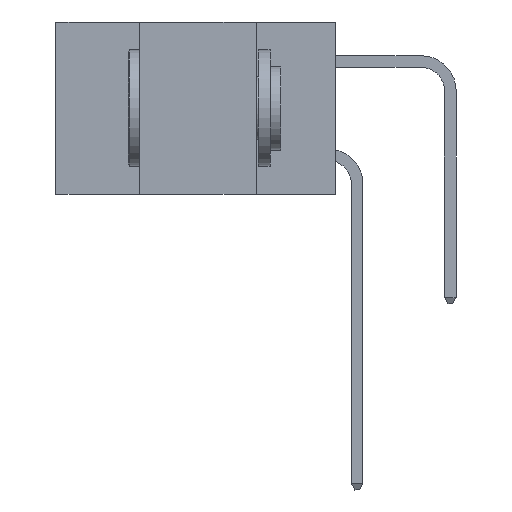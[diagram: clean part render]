
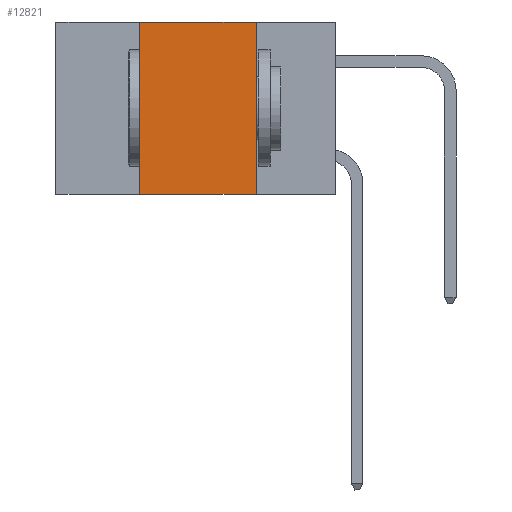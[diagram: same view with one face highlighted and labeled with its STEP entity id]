
A CAD part, left-side view. The second image highlights one B-rep face of the part: STEP entity #12821.
In plain terms, the highlighted planar face has unit normal (-1, 0, 0).
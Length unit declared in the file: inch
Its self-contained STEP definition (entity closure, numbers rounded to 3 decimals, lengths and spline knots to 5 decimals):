
#27 = VECTOR ( 'NONE', #1801, 39.37008 ) ;
#395 = PLANE ( 'NONE',  #2905 ) ;
#470 = CARTESIAN_POINT ( 'NONE',  ( 0., 0.17, -0.37 ) ) ;
#529 = VERTEX_POINT ( 'NONE', #3478 ) ;
#554 = CARTESIAN_POINT ( 'NONE',  ( 0., 0.42, 0. ) ) ;
#1751 = CARTESIAN_POINT ( 'NONE',  ( 0., 0.42, 0. ) ) ;
#1801 = DIRECTION ( 'NONE',  ( 0., 0., 1. ) ) ;
#2308 = CARTESIAN_POINT ( 'NONE',  ( 0., 0.17, 0. ) ) ;
#2494 = ORIENTED_EDGE ( 'NONE', *, *, #14332, .F. ) ;
#2875 = DIRECTION ( 'NONE',  ( 0., 0., -1. ) ) ;
#2905 = AXIS2_PLACEMENT_3D ( 'NONE', #9037, #10246, #2875 ) ;
#3236 = ORIENTED_EDGE ( 'NONE', *, *, #7011, .F. ) ;
#3435 = ORIENTED_EDGE ( 'NONE', *, *, #10594, .F. ) ;
#3454 = ORIENTED_EDGE ( 'NONE', *, *, #12549, .T. ) ;
#3478 = CARTESIAN_POINT ( 'NONE',  ( 0., 0.42, -0.37 ) ) ;
#5874 = DIRECTION ( 'NONE',  ( 0., -1., 0. ) ) ;
#5983 = VERTEX_POINT ( 'NONE', #13026 ) ;
#6035 = DIRECTION ( 'NONE',  ( 0., 0., -1. ) ) ;
#7011 = EDGE_CURVE ( 'NONE', #12459, #5983, #14390, .T. ) ;
#7764 = VECTOR ( 'NONE', #6035, 39.37008 ) ;
#9037 = CARTESIAN_POINT ( 'NONE',  ( 0., 0.6, 0. ) ) ;
#9302 = CARTESIAN_POINT ( 'NONE',  ( 0., 0.6, -0.37 ) ) ;
#9838 = LINE ( 'NONE', #554, #27 ) ;
#10246 = DIRECTION ( 'NONE',  ( 1., 0., 0. ) ) ;
#10343 = VECTOR ( 'NONE', #10521, 39.37008 ) ;
#10521 = DIRECTION ( 'NONE',  ( 0., -1., 0. ) ) ;
#10594 = EDGE_CURVE ( 'NONE', #529, #12459, #9838, .T. ) ;
#10742 = CARTESIAN_POINT ( 'NONE',  ( 0., 0.6, 0. ) ) ;
#11086 = VECTOR ( 'NONE', #5874, 39.37008 ) ;
#11842 = EDGE_LOOP ( 'NONE', ( #2494, #3236, #3435, #3454 ) ) ;
#11891 = FACE_OUTER_BOUND ( 'NONE', #11842, .T. ) ;
#12459 = VERTEX_POINT ( 'NONE', #1751 ) ;
#12549 = EDGE_CURVE ( 'NONE', #529, #14020, #14040, .T. ) ;
#12821 = ADVANCED_FACE ( 'NONE', ( #11891 ), #395, .F. ) ;
#13026 = CARTESIAN_POINT ( 'NONE',  ( 0., 0.17, 0. ) ) ;
#14020 = VERTEX_POINT ( 'NONE', #470 ) ;
#14040 = LINE ( 'NONE', #9302, #10343 ) ;
#14326 = LINE ( 'NONE', #2308, #7764 ) ;
#14332 = EDGE_CURVE ( 'NONE', #5983, #14020, #14326, .T. ) ;
#14390 = LINE ( 'NONE', #10742, #11086 ) ;
